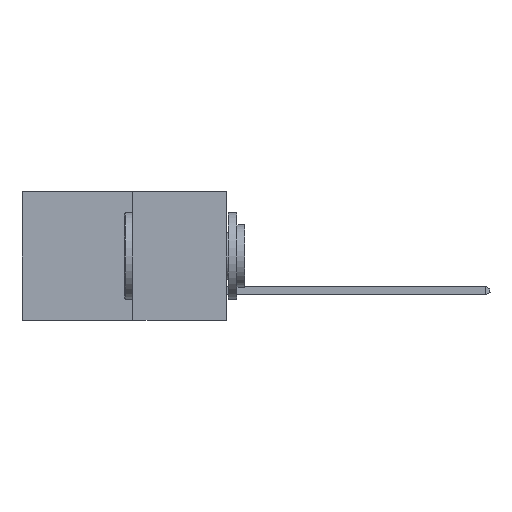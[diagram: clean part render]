
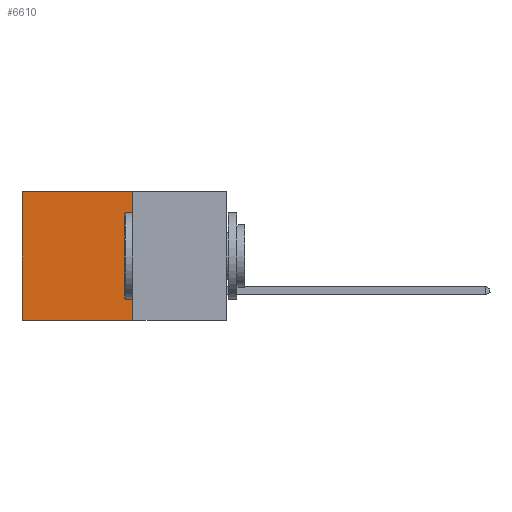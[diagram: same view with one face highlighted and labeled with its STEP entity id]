
A CAD part, left-side view. The second image highlights one B-rep face of the part: STEP entity #6610.
In plain terms, the highlighted planar face has unit normal (-1, 0, 0).
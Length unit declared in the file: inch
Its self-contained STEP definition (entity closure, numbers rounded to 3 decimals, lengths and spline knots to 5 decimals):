
#489 = EDGE_LOOP ( 'NONE', ( #2820, #15578, #14318, #9025 ) ) ;
#990 = CARTESIAN_POINT ( 'NONE',  ( 0.277, 0.59, 0. ) ) ;
#1167 = LINE ( 'NONE', #14179, #8221 ) ;
#2820 = ORIENTED_EDGE ( 'NONE', *, *, #14299, .T. ) ;
#3584 = CARTESIAN_POINT ( 'NONE',  ( 0.277, 0.27, 0. ) ) ;
#4290 = VECTOR ( 'NONE', #4739, 39.37008 ) ;
#4672 = AXIS2_PLACEMENT_3D ( 'NONE', #15461, #15435, #15432 ) ;
#4708 = VECTOR ( 'NONE', #4813, 39.37008 ) ;
#4739 = DIRECTION ( 'NONE',  ( 0., 0., -1. ) ) ;
#4813 = DIRECTION ( 'NONE',  ( 0., 1., 0. ) ) ;
#5095 = LINE ( 'NONE', #11516, #4708 ) ;
#5203 = CARTESIAN_POINT ( 'NONE',  ( 0.277, 0.59, -0.37 ) ) ;
#5537 = VERTEX_POINT ( 'NONE', #5203 ) ;
#5567 = FACE_OUTER_BOUND ( 'NONE', #489, .T. ) ;
#6004 = CARTESIAN_POINT ( 'NONE',  ( 0.277, 0.59, -0.37 ) ) ;
#6146 = DIRECTION ( 'NONE',  ( 0., 0., -1. ) ) ;
#6164 = CARTESIAN_POINT ( 'NONE',  ( 0.277, 0.27, -0.37 ) ) ;
#6209 = EDGE_CURVE ( 'NONE', #8126, #10049, #8355, .T. ) ;
#6610 = ADVANCED_FACE ( 'NONE', ( #5567 ), #15483, .F. ) ;
#8126 = VERTEX_POINT ( 'NONE', #3584 ) ;
#8221 = VECTOR ( 'NONE', #14043, 39.37008 ) ;
#8355 = LINE ( 'NONE', #6164, #15731 ) ;
#9025 = ORIENTED_EDGE ( 'NONE', *, *, #9891, .T. ) ;
#9891 = EDGE_CURVE ( 'NONE', #8126, #11706, #1167, .T. ) ;
#10049 = VERTEX_POINT ( 'NONE', #12533 ) ;
#11516 = CARTESIAN_POINT ( 'NONE',  ( 0.277, 0.27, -0.37 ) ) ;
#11706 = VERTEX_POINT ( 'NONE', #990 ) ;
#11849 = LINE ( 'NONE', #6004, #4290 ) ;
#12533 = CARTESIAN_POINT ( 'NONE',  ( 0.277, 0.27, -0.37 ) ) ;
#13597 = EDGE_CURVE ( 'NONE', #10049, #5537, #5095, .T. ) ;
#14043 = DIRECTION ( 'NONE',  ( 0., 1., 0. ) ) ;
#14179 = CARTESIAN_POINT ( 'NONE',  ( 0.277, 0.27, 0. ) ) ;
#14299 = EDGE_CURVE ( 'NONE', #11706, #5537, #11849, .T. ) ;
#14318 = ORIENTED_EDGE ( 'NONE', *, *, #6209, .F. ) ;
#15432 = DIRECTION ( 'NONE',  ( 0., 0., -1. ) ) ;
#15435 = DIRECTION ( 'NONE',  ( 1., 0., 0. ) ) ;
#15461 = CARTESIAN_POINT ( 'NONE',  ( 0.277, 0.27, -0.37 ) ) ;
#15483 = PLANE ( 'NONE',  #4672 ) ;
#15578 = ORIENTED_EDGE ( 'NONE', *, *, #13597, .F. ) ;
#15731 = VECTOR ( 'NONE', #6146, 39.37008 ) ;
